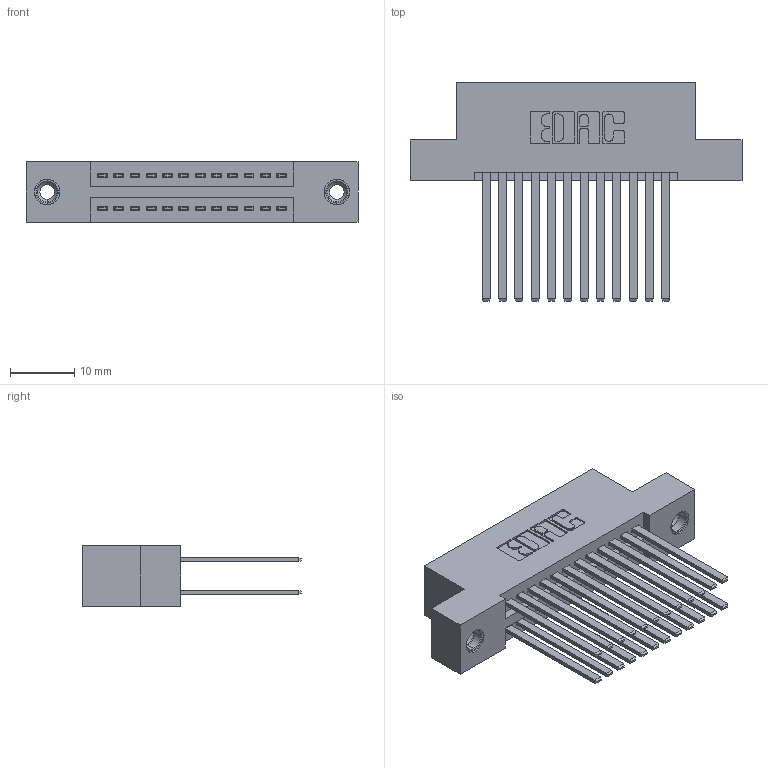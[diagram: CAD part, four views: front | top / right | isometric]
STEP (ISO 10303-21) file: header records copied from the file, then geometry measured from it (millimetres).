
FILE_DESCRIPTION (( 'STEP AP203' ), '1' );
FILE_NAME ('345-024-544-208.STEP', '2019-10-27T17:21:04', ( '' ), ( '' ), 'SwSTEP 2.0', 'SolidWorks 2016', '' );
FILE_SCHEMA (( 'CONFIG_CONTROL_DESIGN' ));
Length unit declared in the file: inch
Products named in the file (4): 345-250-001_345-250-003-102; 345 Part_Flush Mounting Lugs - 0.156 Dia-TI; 345-024-544-208; 345-292-001_345-293-144
Assembly tree (27 placements, depth 2):
  345-024-544-208
    345 Part_Flush Mounting Lugs - 0.156 Dia-TI
    345-292-001_345-293-144  x24
    345-250-001_345-250-003-102  x2
Bounding box: 51.69 x 33.96 x 9.4 mm (x, y, z)
Volume: 5072.6 mm3; surface area: 7916.6 mm2
Topology: 27 solids, 27 shells, 1242 faces, 3621 edges, 2374 vertices
Faces by surface type: plane 808, cylinder 418, cone 12, torus 4
Entity records: 14456 total; most frequent: CARTESIAN_POINT 2431, ORIENTED_EDGE 2358, DIRECTION 2205, EDGE_CURVE 1179, LINE 983, VECTOR 983, VERTEX_POINT 780, AXIS2_PLACEMENT_3D 611
